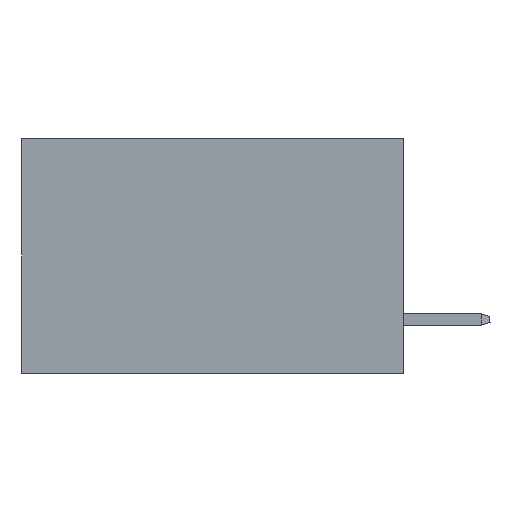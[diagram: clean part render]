
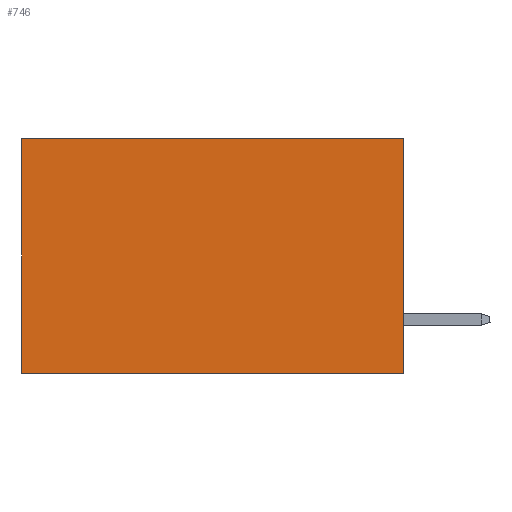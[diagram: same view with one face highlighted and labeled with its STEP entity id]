
A CAD part, left-side view. The second image highlights one B-rep face of the part: STEP entity #746.
In plain terms, the highlighted planar face has unit normal (-1, 0, 0).
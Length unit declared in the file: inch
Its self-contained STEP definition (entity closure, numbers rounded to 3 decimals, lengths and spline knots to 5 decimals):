
#746 = ADVANCED_FACE ( 'NONE', ( #26496 ), #9021, .F. ) ;
#937 = VERTEX_POINT ( 'NONE', #21416 ) ;
#4620 = CARTESIAN_POINT ( 'NONE',  ( 0.2875, 0., 0. ) ) ;
#5291 = CARTESIAN_POINT ( 'NONE',  ( 0.2875, 0., 0. ) ) ;
#5418 = VECTOR ( 'NONE', #39006, 39.37008 ) ;
#5477 = EDGE_CURVE ( 'NONE', #21109, #937, #25365, .T. ) ;
#6716 = DIRECTION ( 'NONE',  ( 0., 1., 0. ) ) ;
#8589 = CARTESIAN_POINT ( 'NONE',  ( 0.2875, 0., 0. ) ) ;
#9021 = PLANE ( 'NONE',  #35717 ) ;
#9842 = CARTESIAN_POINT ( 'NONE',  ( 0.2875, 0., -0.37 ) ) ;
#11578 = LINE ( 'NONE', #8589, #12602 ) ;
#12602 = VECTOR ( 'NONE', #44097, 39.37008 ) ;
#17302 = LINE ( 'NONE', #38334, #23236 ) ;
#17311 = EDGE_CURVE ( 'NONE', #39831, #937, #17302, .T. ) ;
#18908 = DIRECTION ( 'NONE',  ( 1., 0., 0. ) ) ;
#19350 = DIRECTION ( 'NONE',  ( 0., 0., -1. ) ) ;
#21109 = VERTEX_POINT ( 'NONE', #39610 ) ;
#21416 = CARTESIAN_POINT ( 'NONE',  ( 0.2875, 0.6, -0.37 ) ) ;
#23171 = ORIENTED_EDGE ( 'NONE', *, *, #5477, .T. ) ;
#23236 = VECTOR ( 'NONE', #6716, 39.37008 ) ;
#25365 = LINE ( 'NONE', #43371, #5418 ) ;
#26262 = LINE ( 'NONE', #5291, #34426 ) ;
#26496 = FACE_OUTER_BOUND ( 'NONE', #39211, .T. ) ;
#26651 = VERTEX_POINT ( 'NONE', #34573 ) ;
#33003 = DIRECTION ( 'NONE',  ( 0., 0., -1. ) ) ;
#34426 = VECTOR ( 'NONE', #19350, 39.37008 ) ;
#34573 = CARTESIAN_POINT ( 'NONE',  ( 0.2875, 0., 0. ) ) ;
#34846 = ORIENTED_EDGE ( 'NONE', *, *, #43929, .T. ) ;
#35129 = ORIENTED_EDGE ( 'NONE', *, *, #38135, .F. ) ;
#35717 = AXIS2_PLACEMENT_3D ( 'NONE', #4620, #18908, #33003 ) ;
#38135 = EDGE_CURVE ( 'NONE', #26651, #39831, #26262, .T. ) ;
#38334 = CARTESIAN_POINT ( 'NONE',  ( 0.2875, 0., -0.37 ) ) ;
#39006 = DIRECTION ( 'NONE',  ( 0., 0., -1. ) ) ;
#39211 = EDGE_LOOP ( 'NONE', ( #23171, #41348, #35129, #34846 ) ) ;
#39610 = CARTESIAN_POINT ( 'NONE',  ( 0.2875, 0.6, 0. ) ) ;
#39831 = VERTEX_POINT ( 'NONE', #9842 ) ;
#41348 = ORIENTED_EDGE ( 'NONE', *, *, #17311, .F. ) ;
#43371 = CARTESIAN_POINT ( 'NONE',  ( 0.2875, 0.6, 0. ) ) ;
#43929 = EDGE_CURVE ( 'NONE', #26651, #21109, #11578, .T. ) ;
#44097 = DIRECTION ( 'NONE',  ( 0., 1., 0. ) ) ;
